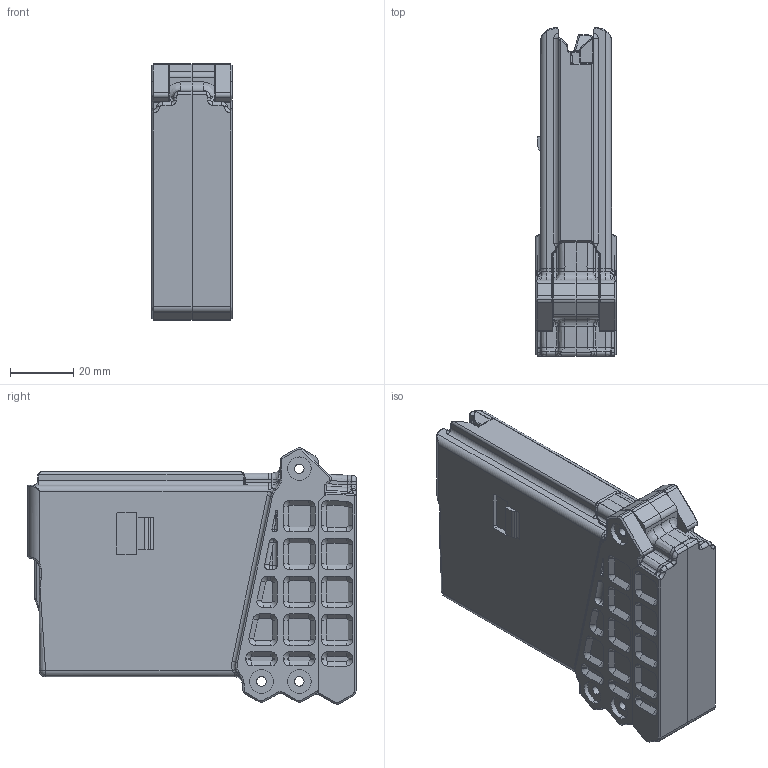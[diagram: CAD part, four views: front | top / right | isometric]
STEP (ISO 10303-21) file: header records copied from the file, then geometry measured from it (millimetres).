
FILE_DESCRIPTION (( 'STEP AP214' ), '1' );
FILE_NAME ('Ten Round Magazine.STEP', '2021-05-01T22:56:51', ( '' ), ( '' ), 'SwSTEP 2.0', 'SolidWorks 2020', '' );
FILE_SCHEMA (( 'AUTOMOTIVE_DESIGN' ));
Length unit declared in the file: millimetre
Products named in the file (5): Ten Round Magazine; Ten Round Mag Body Bottom Right; Mag Follower; Mag Body Top; Ten Round Mag Body Bottom Left
Assembly tree (4 placements, depth 2):
  Ten Round Magazine
    Mag Body Top
    Mag Follower
    Ten Round Mag Body Bottom Right
    Ten Round Mag Body Bottom Left
Bounding box: 25.5 x 104 x 81.23 mm (x, y, z)
Volume: 63211.9 mm3; surface area: 48200 mm2
Topology: 4 solids, 4 shells, 1787 faces, 4611 edges, 2792 vertices
Faces by surface type: cylinder 561, plane 471, bspline 446, cone 152, torus 126, sphere 31
Entity records: 68201 total; most frequent: CARTESIAN_POINT 28510, ORIENTED_EDGE 9046, DIRECTION 7350, EDGE_CURVE 4523, VERTEX_POINT 2785, AXIS2_PLACEMENT_3D 2761, EDGE_LOOP 1858, LINE 1828
